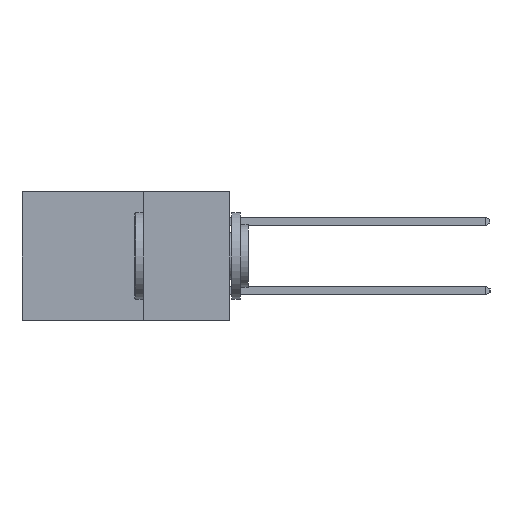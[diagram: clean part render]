
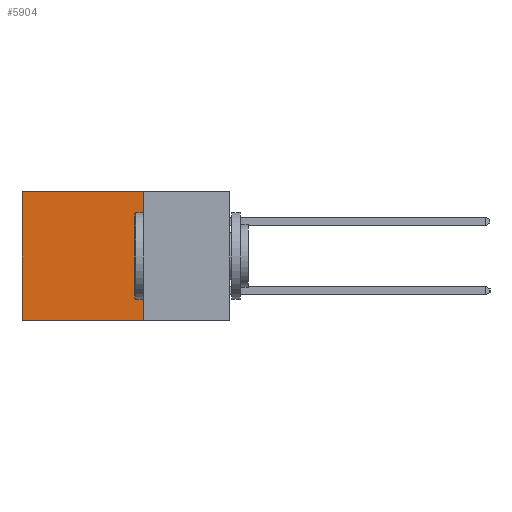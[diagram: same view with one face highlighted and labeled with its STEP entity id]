
A CAD part, left-side view. The second image highlights one B-rep face of the part: STEP entity #5904.
In plain terms, the highlighted planar face has unit normal (-1, 0, 0).
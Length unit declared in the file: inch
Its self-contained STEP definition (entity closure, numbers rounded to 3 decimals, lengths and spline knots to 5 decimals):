
#396 = CARTESIAN_POINT ( 'NONE',  ( 0.2615, 0.25, -0.37 ) ) ;
#827 = LINE ( 'NONE', #3026, #7607 ) ;
#1163 = AXIS2_PLACEMENT_3D ( 'NONE', #396, #6823, #1299 ) ;
#1299 = DIRECTION ( 'NONE',  ( 0., 0., -1. ) ) ;
#1480 = CARTESIAN_POINT ( 'NONE',  ( 0.2615, 0.25, -0.37 ) ) ;
#2884 = EDGE_CURVE ( 'NONE', #4774, #7410, #4099, .T. ) ;
#3026 = CARTESIAN_POINT ( 'NONE',  ( 0.2615, 0.25, -0.37 ) ) ;
#3483 = VERTEX_POINT ( 'NONE', #1480 ) ;
#3814 = VECTOR ( 'NONE', #9051, 39.37008 ) ;
#3847 = DIRECTION ( 'NONE',  ( 0., 0., -1. ) ) ;
#3944 = ORIENTED_EDGE ( 'NONE', *, *, #6554, .F. ) ;
#4037 = ORIENTED_EDGE ( 'NONE', *, *, #2884, .T. ) ;
#4099 = LINE ( 'NONE', #9949, #3814 ) ;
#4757 = CARTESIAN_POINT ( 'NONE',  ( 0.2615, 0.6, -0.37 ) ) ;
#4774 = VERTEX_POINT ( 'NONE', #6942 ) ;
#4981 = CARTESIAN_POINT ( 'NONE',  ( 0.2615, 0.25, -0.37 ) ) ;
#5030 = LINE ( 'NONE', #4981, #7222 ) ;
#5296 = CARTESIAN_POINT ( 'NONE',  ( 0.2615, 0.6, 0. ) ) ;
#5767 = DIRECTION ( 'NONE',  ( 0., 0., -1. ) ) ;
#5904 = ADVANCED_FACE ( 'NONE', ( #6070 ), #6783, .F. ) ;
#6045 = CARTESIAN_POINT ( 'NONE',  ( 0.2615, 0.6, -0.37 ) ) ;
#6070 = FACE_OUTER_BOUND ( 'NONE', #10306, .T. ) ;
#6554 = EDGE_CURVE ( 'NONE', #3483, #9620, #5030, .T. ) ;
#6783 = PLANE ( 'NONE',  #1163 ) ;
#6823 = DIRECTION ( 'NONE',  ( 1., 0., 0. ) ) ;
#6942 = CARTESIAN_POINT ( 'NONE',  ( 0.2615, 0.25, 0. ) ) ;
#7222 = VECTOR ( 'NONE', #10491, 39.37008 ) ;
#7410 = VERTEX_POINT ( 'NONE', #5296 ) ;
#7607 = VECTOR ( 'NONE', #5767, 39.37008 ) ;
#7936 = ORIENTED_EDGE ( 'NONE', *, *, #10028, .T. ) ;
#8339 = ORIENTED_EDGE ( 'NONE', *, *, #8457, .F. ) ;
#8457 = EDGE_CURVE ( 'NONE', #4774, #3483, #827, .T. ) ;
#9032 = VECTOR ( 'NONE', #3847, 39.37008 ) ;
#9051 = DIRECTION ( 'NONE',  ( 0., 1., 0. ) ) ;
#9620 = VERTEX_POINT ( 'NONE', #6045 ) ;
#9949 = CARTESIAN_POINT ( 'NONE',  ( 0.2615, 0.25, 0. ) ) ;
#10028 = EDGE_CURVE ( 'NONE', #7410, #9620, #11381, .T. ) ;
#10306 = EDGE_LOOP ( 'NONE', ( #7936, #3944, #8339, #4037 ) ) ;
#10491 = DIRECTION ( 'NONE',  ( 0., 1., 0. ) ) ;
#11381 = LINE ( 'NONE', #4757, #9032 ) ;
